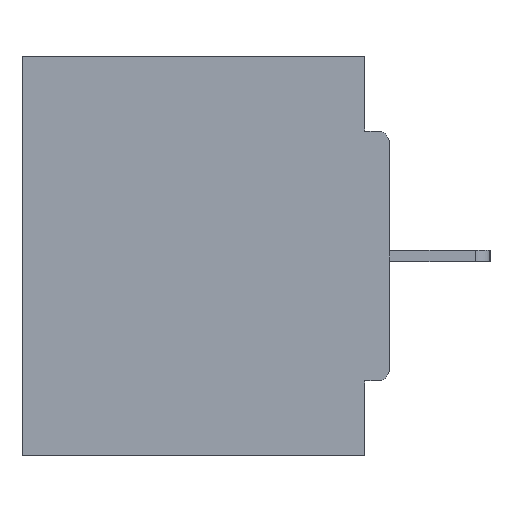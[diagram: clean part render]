
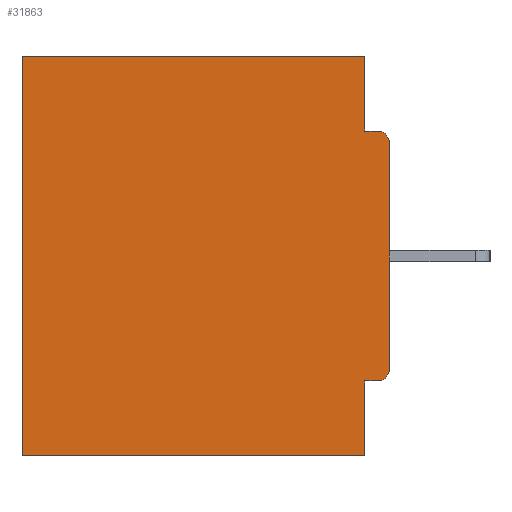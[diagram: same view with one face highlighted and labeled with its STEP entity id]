
A CAD part, left-side view. The second image highlights one B-rep face of the part: STEP entity #31863.
In plain terms, the highlighted planar face has unit normal (-1, 0, 0).
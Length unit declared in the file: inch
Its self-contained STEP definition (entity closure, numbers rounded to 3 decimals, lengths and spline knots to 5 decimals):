
#634 = VECTOR ( 'NONE', #29605, 39.37008 ) ;
#646 = CARTESIAN_POINT ( 'NONE',  ( 0.298, 0., 0. ) ) ;
#1301 = ORIENTED_EDGE ( 'NONE', *, *, #5563, .F. ) ;
#1569 = CARTESIAN_POINT ( 'NONE',  ( 0.298, 0., -0.3915 ) ) ;
#1657 = LINE ( 'NONE', #12977, #28913 ) ;
#1807 = LINE ( 'NONE', #646, #13596 ) ;
#1869 = CARTESIAN_POINT ( 'NONE',  ( 0.298, 0.015, -0.1085 ) ) ;
#2889 = EDGE_CURVE ( 'NONE', #10276, #7726, #27442, .T. ) ;
#3129 = ORIENTED_EDGE ( 'NONE', *, *, #8782, .F. ) ;
#3681 = VERTEX_POINT ( 'NONE', #13172 ) ;
#4464 = DIRECTION ( 'NONE',  ( 0., 0., -1. ) ) ;
#4582 = DIRECTION ( 'NONE',  ( -1., 0., 0. ) ) ;
#4590 = DIRECTION ( 'NONE',  ( 0., 0., -1. ) ) ;
#4591 = CARTESIAN_POINT ( 'NONE',  ( 0.298, 0.015, -0.3915 ) ) ;
#4761 = LINE ( 'NONE', #28942, #18148 ) ;
#4784 = VERTEX_POINT ( 'NONE', #33225 ) ;
#4905 = CARTESIAN_POINT ( 'NONE',  ( 0.298, 0., -0.5 ) ) ;
#5563 = EDGE_CURVE ( 'NONE', #10953, #7726, #9267, .T. ) ;
#7628 = DIRECTION ( 'NONE',  ( 0., 1., 0. ) ) ;
#7726 = VERTEX_POINT ( 'NONE', #1569 ) ;
#7839 = LINE ( 'NONE', #24477, #634 ) ;
#8229 = ORIENTED_EDGE ( 'NONE', *, *, #19817, .F. ) ;
#8411 = VECTOR ( 'NONE', #33901, 39.37008 ) ;
#8782 = EDGE_CURVE ( 'NONE', #10276, #4784, #4761, .T. ) ;
#8846 = VECTOR ( 'NONE', #7628, 39.37008 ) ;
#9098 = AXIS2_PLACEMENT_3D ( 'NONE', #17676, #28104, #12482 ) ;
#9267 = LINE ( 'NONE', #33339, #8411 ) ;
#9587 = VECTOR ( 'NONE', #14181, 39.37008 ) ;
#10276 = VERTEX_POINT ( 'NONE', #11985 ) ;
#10953 = VERTEX_POINT ( 'NONE', #32845 ) ;
#11985 = CARTESIAN_POINT ( 'NONE',  ( 0.298, 0.015, -0.4065 ) ) ;
#12244 = EDGE_CURVE ( 'NONE', #22513, #16424, #30481, .T. ) ;
#12482 = DIRECTION ( 'NONE',  ( 0., 0., -1. ) ) ;
#12977 = CARTESIAN_POINT ( 'NONE',  ( 0.298, 0.46, 0. ) ) ;
#13172 = CARTESIAN_POINT ( 'NONE',  ( 0.298, 0.031, -0.0935 ) ) ;
#13596 = VECTOR ( 'NONE', #19486, 39.37008 ) ;
#13598 = ORIENTED_EDGE ( 'NONE', *, *, #25162, .F. ) ;
#13893 = VERTEX_POINT ( 'NONE', #17184 ) ;
#14023 = CARTESIAN_POINT ( 'NONE',  ( 0.298, 0.46, 0. ) ) ;
#14181 = DIRECTION ( 'NONE',  ( 0., 0., -1. ) ) ;
#15029 = ORIENTED_EDGE ( 'NONE', *, *, #32239, .T. ) ;
#15124 = ORIENTED_EDGE ( 'NONE', *, *, #2889, .T. ) ;
#16093 = CARTESIAN_POINT ( 'NONE',  ( 0.298, 0., -0.0935 ) ) ;
#16385 = DIRECTION ( 'NONE',  ( 0., 1., 0. ) ) ;
#16424 = VERTEX_POINT ( 'NONE', #19992 ) ;
#16583 = LINE ( 'NONE', #16093, #22729 ) ;
#16592 = CIRCLE ( 'NONE', #27731, 0.015 ) ;
#16817 = CARTESIAN_POINT ( 'NONE',  ( 0.298, 0.031, -0.5 ) ) ;
#17184 = CARTESIAN_POINT ( 'NONE',  ( 0.298, 0.031, 0. ) ) ;
#17462 = VERTEX_POINT ( 'NONE', #19128 ) ;
#17676 = CARTESIAN_POINT ( 'NONE',  ( 0.298, 0., 0. ) ) ;
#18148 = VECTOR ( 'NONE', #16385, 39.37008 ) ;
#19128 = CARTESIAN_POINT ( 'NONE',  ( 0.298, 0.015, -0.0935 ) ) ;
#19486 = DIRECTION ( 'NONE',  ( 0., 1., 0. ) ) ;
#19556 = EDGE_LOOP ( 'NONE', ( #24747, #25805, #8229, #15029, #30008, #28737, #13598, #3129, #15124, #1301 ) ) ;
#19817 = EDGE_CURVE ( 'NONE', #13893, #3681, #31145, .T. ) ;
#19992 = CARTESIAN_POINT ( 'NONE',  ( 0.298, 0.46, -0.5 ) ) ;
#20277 = EDGE_CURVE ( 'NONE', #3681, #17462, #16583, .T. ) ;
#20537 = DIRECTION ( 'NONE',  ( -1., 0., 0. ) ) ;
#20894 = DIRECTION ( 'NONE',  ( 0., 0., -1. ) ) ;
#22513 = VERTEX_POINT ( 'NONE', #22829 ) ;
#22729 = VECTOR ( 'NONE', #31535, 39.37008 ) ;
#22829 = CARTESIAN_POINT ( 'NONE',  ( 0.298, 0.031, -0.5 ) ) ;
#24041 = VERTEX_POINT ( 'NONE', #14023 ) ;
#24477 = CARTESIAN_POINT ( 'NONE',  ( 0.298, 0.031, -0.5 ) ) ;
#24716 = AXIS2_PLACEMENT_3D ( 'NONE', #4591, #4582, #4464 ) ;
#24747 = ORIENTED_EDGE ( 'NONE', *, *, #30116, .T. ) ;
#25162 = EDGE_CURVE ( 'NONE', #4784, #22513, #7839, .T. ) ;
#25526 = PLANE ( 'NONE',  #9098 ) ;
#25805 = ORIENTED_EDGE ( 'NONE', *, *, #20277, .F. ) ;
#27442 = CIRCLE ( 'NONE', #24716, 0.015 ) ;
#27731 = AXIS2_PLACEMENT_3D ( 'NONE', #1869, #20537, #4590 ) ;
#28104 = DIRECTION ( 'NONE',  ( 1., 0., 0. ) ) ;
#28737 = ORIENTED_EDGE ( 'NONE', *, *, #12244, .F. ) ;
#28913 = VECTOR ( 'NONE', #20894, 39.37008 ) ;
#28942 = CARTESIAN_POINT ( 'NONE',  ( 0.298, 0., -0.4065 ) ) ;
#29605 = DIRECTION ( 'NONE',  ( 0., 0., -1. ) ) ;
#30008 = ORIENTED_EDGE ( 'NONE', *, *, #32778, .T. ) ;
#30116 = EDGE_CURVE ( 'NONE', #10953, #17462, #16592, .T. ) ;
#30481 = LINE ( 'NONE', #4905, #8846 ) ;
#31145 = LINE ( 'NONE', #16817, #9587 ) ;
#31535 = DIRECTION ( 'NONE',  ( 0., -1., 0. ) ) ;
#31863 = ADVANCED_FACE ( 'NONE', ( #33402 ), #25526, .F. ) ;
#32239 = EDGE_CURVE ( 'NONE', #13893, #24041, #1807, .T. ) ;
#32778 = EDGE_CURVE ( 'NONE', #24041, #16424, #1657, .T. ) ;
#32845 = CARTESIAN_POINT ( 'NONE',  ( 0.298, 0., -0.1085 ) ) ;
#33225 = CARTESIAN_POINT ( 'NONE',  ( 0.298, 0.031, -0.4065 ) ) ;
#33339 = CARTESIAN_POINT ( 'NONE',  ( 0.298, 0., 0. ) ) ;
#33402 = FACE_OUTER_BOUND ( 'NONE', #19556, .T. ) ;
#33901 = DIRECTION ( 'NONE',  ( 0., 0., -1. ) ) ;
